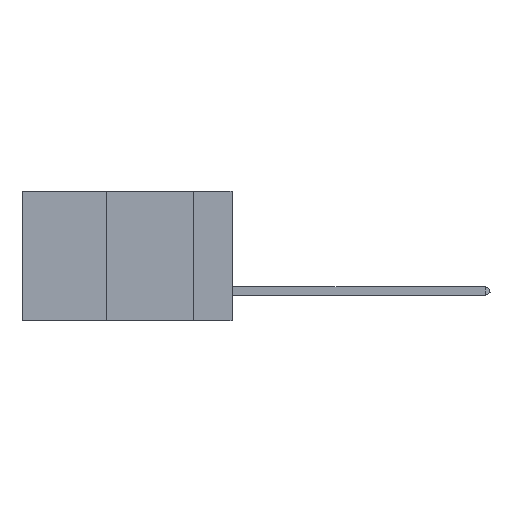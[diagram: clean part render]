
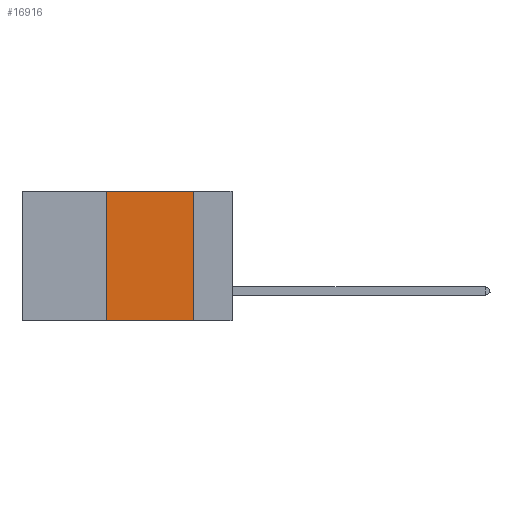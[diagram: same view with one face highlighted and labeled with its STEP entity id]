
A CAD part, left-side view. The second image highlights one B-rep face of the part: STEP entity #16916.
In plain terms, the highlighted planar face has unit normal (-1, 0, 0).
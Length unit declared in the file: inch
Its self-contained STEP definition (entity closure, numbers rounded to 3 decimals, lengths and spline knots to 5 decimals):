
#79 = ORIENTED_EDGE ( 'NONE', *, *, #17444, .F. ) ;
#122 = CARTESIAN_POINT ( 'NONE',  ( 0., 0.36, 0. ) ) ;
#1794 = VECTOR ( 'NONE', #35345, 39.37008 ) ;
#2723 = EDGE_CURVE ( 'NONE', #20511, #22865, #28104, .T. ) ;
#6409 = CARTESIAN_POINT ( 'NONE',  ( 0., 0.6, -0.37 ) ) ;
#7754 = CARTESIAN_POINT ( 'NONE',  ( 0., 0.6, 0. ) ) ;
#8723 = ORIENTED_EDGE ( 'NONE', *, *, #31605, .F. ) ;
#10211 = ORIENTED_EDGE ( 'NONE', *, *, #2723, .T. ) ;
#10289 = DIRECTION ( 'NONE',  ( 1., 0., 0. ) ) ;
#11620 = CARTESIAN_POINT ( 'NONE',  ( 0., 0.11, -0.37 ) ) ;
#11848 = DIRECTION ( 'NONE',  ( 0., -1., 0. ) ) ;
#11897 = CARTESIAN_POINT ( 'NONE',  ( 0., 0.36, 0. ) ) ;
#16540 = LINE ( 'NONE', #122, #21113 ) ;
#16557 = LINE ( 'NONE', #32828, #1794 ) ;
#16713 = VECTOR ( 'NONE', #24696, 39.37008 ) ;
#16916 = ADVANCED_FACE ( 'NONE', ( #29788 ), #26887, .F. ) ;
#17444 = EDGE_CURVE ( 'NONE', #20511, #25124, #16540, .T. ) ;
#18728 = LINE ( 'NONE', #23984, #16713 ) ;
#18867 = ORIENTED_EDGE ( 'NONE', *, *, #20322, .F. ) ;
#20322 = EDGE_CURVE ( 'NONE', #25124, #28753, #16557, .T. ) ;
#20511 = VERTEX_POINT ( 'NONE', #33195 ) ;
#21113 = VECTOR ( 'NONE', #24845, 39.37008 ) ;
#22865 = VERTEX_POINT ( 'NONE', #11620 ) ;
#23570 = CARTESIAN_POINT ( 'NONE',  ( 0., 0.11, 0. ) ) ;
#23954 = AXIS2_PLACEMENT_3D ( 'NONE', #7754, #10289, #29970 ) ;
#23984 = CARTESIAN_POINT ( 'NONE',  ( 0., 0.11, 0. ) ) ;
#24696 = DIRECTION ( 'NONE',  ( 0., 0., -1. ) ) ;
#24845 = DIRECTION ( 'NONE',  ( 0., 0., 1. ) ) ;
#25124 = VERTEX_POINT ( 'NONE', #11897 ) ;
#26887 = PLANE ( 'NONE',  #23954 ) ;
#28104 = LINE ( 'NONE', #6409, #29444 ) ;
#28753 = VERTEX_POINT ( 'NONE', #23570 ) ;
#29444 = VECTOR ( 'NONE', #11848, 39.37008 ) ;
#29788 = FACE_OUTER_BOUND ( 'NONE', #30116, .T. ) ;
#29970 = DIRECTION ( 'NONE',  ( 0., 0., -1. ) ) ;
#30116 = EDGE_LOOP ( 'NONE', ( #8723, #18867, #79, #10211 ) ) ;
#31605 = EDGE_CURVE ( 'NONE', #28753, #22865, #18728, .T. ) ;
#32828 = CARTESIAN_POINT ( 'NONE',  ( 0., 0.6, 0. ) ) ;
#33195 = CARTESIAN_POINT ( 'NONE',  ( 0., 0.36, -0.37 ) ) ;
#35345 = DIRECTION ( 'NONE',  ( 0., -1., 0. ) ) ;
